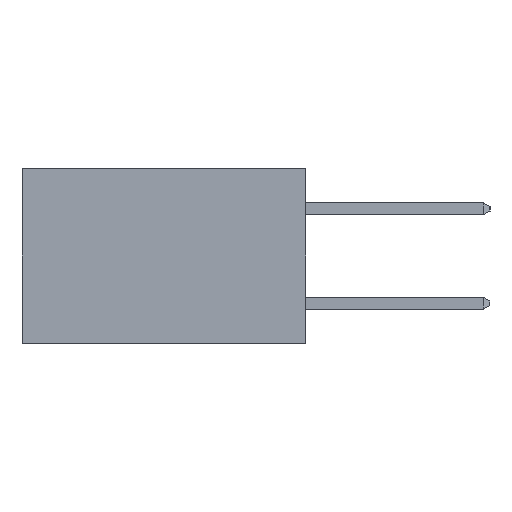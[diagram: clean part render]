
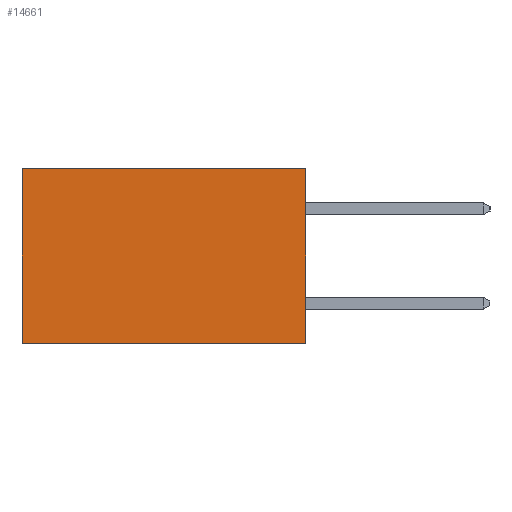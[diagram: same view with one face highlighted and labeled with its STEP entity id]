
A CAD part, left-side view. The second image highlights one B-rep face of the part: STEP entity #14661.
In plain terms, the highlighted planar face has unit normal (-1, 0, 0).
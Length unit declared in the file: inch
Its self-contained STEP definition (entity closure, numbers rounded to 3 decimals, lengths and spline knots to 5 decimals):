
#236 = ORIENTED_EDGE ( 'NONE', *, *, #7093, .T. ) ;
#1030 = AXIS2_PLACEMENT_3D ( 'NONE', #7502, #14718, #6094 ) ;
#1690 = LINE ( 'NONE', #16689, #8993 ) ;
#2611 = VECTOR ( 'NONE', #3164, 39.37008 ) ;
#3164 = DIRECTION ( 'NONE',  ( 0., 0., -1. ) ) ;
#3548 = VERTEX_POINT ( 'NONE', #7290 ) ;
#4424 = CARTESIAN_POINT ( 'NONE',  ( 0.298, 0., 0. ) ) ;
#4619 = PLANE ( 'NONE',  #1030 ) ;
#5337 = CARTESIAN_POINT ( 'NONE',  ( 0.298, 0.6, 0. ) ) ;
#5474 = CARTESIAN_POINT ( 'NONE',  ( 0.298, 0., -0.37 ) ) ;
#5481 = LINE ( 'NONE', #10448, #16108 ) ;
#5618 = LINE ( 'NONE', #13281, #2611 ) ;
#6033 = EDGE_LOOP ( 'NONE', ( #236, #6444, #13682, #6824 ) ) ;
#6094 = DIRECTION ( 'NONE',  ( 0., 0., -1. ) ) ;
#6444 = ORIENTED_EDGE ( 'NONE', *, *, #10646, .F. ) ;
#6824 = ORIENTED_EDGE ( 'NONE', *, *, #14921, .T. ) ;
#7093 = EDGE_CURVE ( 'NONE', #8799, #17151, #5481, .T. ) ;
#7290 = CARTESIAN_POINT ( 'NONE',  ( 0.298, 0., -0.37 ) ) ;
#7502 = CARTESIAN_POINT ( 'NONE',  ( 0.298, 0., 0. ) ) ;
#8378 = DIRECTION ( 'NONE',  ( 0., 1., 0. ) ) ;
#8799 = VERTEX_POINT ( 'NONE', #5337 ) ;
#8993 = VECTOR ( 'NONE', #10905, 39.37008 ) ;
#9401 = VECTOR ( 'NONE', #8378, 39.37008 ) ;
#10448 = CARTESIAN_POINT ( 'NONE',  ( 0.298, 0.6, 0. ) ) ;
#10646 = EDGE_CURVE ( 'NONE', #3548, #17151, #13193, .T. ) ;
#10905 = DIRECTION ( 'NONE',  ( 0., 1., 0. ) ) ;
#11336 = DIRECTION ( 'NONE',  ( 0., 0., -1. ) ) ;
#12135 = VERTEX_POINT ( 'NONE', #4424 ) ;
#13031 = FACE_OUTER_BOUND ( 'NONE', #6033, .T. ) ;
#13193 = LINE ( 'NONE', #5474, #9401 ) ;
#13281 = CARTESIAN_POINT ( 'NONE',  ( 0.298, 0., 0. ) ) ;
#13682 = ORIENTED_EDGE ( 'NONE', *, *, #17450, .F. ) ;
#14661 = ADVANCED_FACE ( 'NONE', ( #13031 ), #4619, .F. ) ;
#14718 = DIRECTION ( 'NONE',  ( 1., 0., 0. ) ) ;
#14921 = EDGE_CURVE ( 'NONE', #12135, #8799, #1690, .T. ) ;
#16108 = VECTOR ( 'NONE', #11336, 39.37008 ) ;
#16689 = CARTESIAN_POINT ( 'NONE',  ( 0.298, 0., 0. ) ) ;
#16935 = CARTESIAN_POINT ( 'NONE',  ( 0.298, 0.6, -0.37 ) ) ;
#17151 = VERTEX_POINT ( 'NONE', #16935 ) ;
#17450 = EDGE_CURVE ( 'NONE', #12135, #3548, #5618, .T. ) ;
